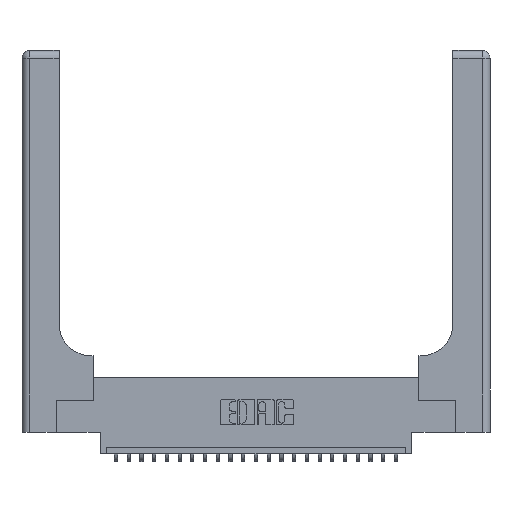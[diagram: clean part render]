
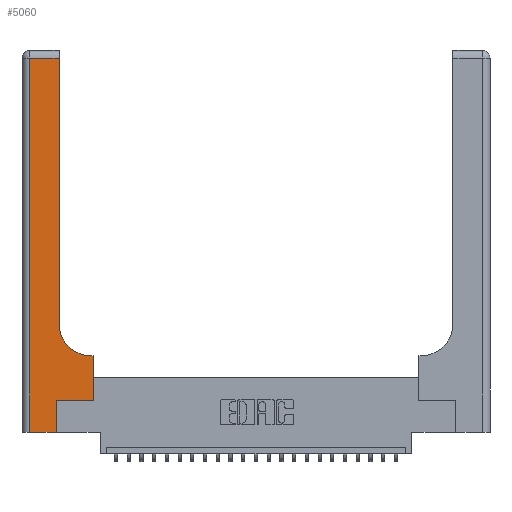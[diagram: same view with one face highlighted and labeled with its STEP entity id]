
A CAD part, top view. The second image highlights one B-rep face of the part: STEP entity #5060.
In plain terms, the highlighted planar face has unit normal (0, 0, 1).
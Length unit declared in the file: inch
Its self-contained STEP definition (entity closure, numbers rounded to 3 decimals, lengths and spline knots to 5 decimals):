
#475 = CARTESIAN_POINT ( 'NONE',  ( 0.269, 0.25, 0.37 ) ) ;
#723 = DIRECTION ( 'NONE',  ( 1., 0., 0. ) ) ;
#1697 = CARTESIAN_POINT ( 'NONE',  ( 0.2915, 3., 0.37 ) ) ;
#2008 = ORIENTED_EDGE ( 'NONE', *, *, #23316, .T. ) ;
#2259 = CARTESIAN_POINT ( 'NONE',  ( 0., 0., 0.37 ) ) ;
#2364 = VERTEX_POINT ( 'NONE', #15380 ) ;
#2484 = EDGE_CURVE ( 'NONE', #16981, #15620, #15268, .T. ) ;
#2587 = VECTOR ( 'NONE', #13204, 39.37008 ) ;
#2593 = LINE ( 'NONE', #14605, #2926 ) ;
#2719 = CARTESIAN_POINT ( 'NONE',  ( 0.06, 3., 0.37 ) ) ;
#2878 = VERTEX_POINT ( 'NONE', #475 ) ;
#2926 = VECTOR ( 'NONE', #5136, 39.37008 ) ;
#3103 = DIRECTION ( 'NONE',  ( -1., 0., 0. ) ) ;
#3133 = DIRECTION ( 'NONE',  ( 0., 0., -1. ) ) ;
#3677 = DIRECTION ( 'NONE',  ( 0., 1., 0. ) ) ;
#3927 = EDGE_CURVE ( 'NONE', #2878, #24777, #5741, .T. ) ;
#4013 = DIRECTION ( 'NONE',  ( -1., 0., 0. ) ) ;
#4089 = VECTOR ( 'NONE', #723, 39.37008 ) ;
#4716 = CARTESIAN_POINT ( 'NONE',  ( 0.06, 2.94, 0.37 ) ) ;
#4819 = AXIS2_PLACEMENT_3D ( 'NONE', #8930, #20790, #3103 ) ;
#5060 = ADVANCED_FACE ( 'NONE', ( #5089 ), #20532, .F. ) ;
#5084 = LINE ( 'NONE', #23223, #7850 ) ;
#5089 = FACE_OUTER_BOUND ( 'NONE', #15781, .T. ) ;
#5136 = DIRECTION ( 'NONE',  ( 0., 1., 0. ) ) ;
#5344 = LINE ( 'NONE', #2259, #4089 ) ;
#5741 = LINE ( 'NONE', #20090, #6657 ) ;
#5994 = VECTOR ( 'NONE', #23192, 39.37008 ) ;
#6182 = EDGE_CURVE ( 'NONE', #15620, #6461, #5344, .T. ) ;
#6461 = VERTEX_POINT ( 'NONE', #20992 ) ;
#6657 = VECTOR ( 'NONE', #23811, 39.37008 ) ;
#6873 = ORIENTED_EDGE ( 'NONE', *, *, #7666, .T. ) ;
#6950 = VERTEX_POINT ( 'NONE', #8498 ) ;
#7040 = CARTESIAN_POINT ( 'NONE',  ( 0.2915, 0.85, 0.37 ) ) ;
#7554 = ORIENTED_EDGE ( 'NONE', *, *, #11364, .T. ) ;
#7666 = EDGE_CURVE ( 'NONE', #19085, #6950, #7728, .T. ) ;
#7728 = LINE ( 'NONE', #1697, #19624 ) ;
#7850 = VECTOR ( 'NONE', #4013, 39.37008 ) ;
#8498 = CARTESIAN_POINT ( 'NONE',  ( 0.2915, 2.94, 0.37 ) ) ;
#8930 = CARTESIAN_POINT ( 'NONE',  ( 0., 3., 0.37 ) ) ;
#9279 = ORIENTED_EDGE ( 'NONE', *, *, #14532, .T. ) ;
#9566 = CARTESIAN_POINT ( 'NONE',  ( 0.269, 0., 0.37 ) ) ;
#10097 = VECTOR ( 'NONE', #18462, 39.37008 ) ;
#11364 = EDGE_CURVE ( 'NONE', #6461, #2878, #21837, .T. ) ;
#11471 = ORIENTED_EDGE ( 'NONE', *, *, #11594, .T. ) ;
#11594 = EDGE_CURVE ( 'NONE', #6950, #16981, #13589, .T. ) ;
#13204 = DIRECTION ( 'NONE',  ( -1., 0., 0. ) ) ;
#13410 = ORIENTED_EDGE ( 'NONE', *, *, #6182, .T. ) ;
#13589 = LINE ( 'NONE', #21007, #2587 ) ;
#14532 = EDGE_CURVE ( 'NONE', #2364, #19539, #5084, .T. ) ;
#14605 = CARTESIAN_POINT ( 'NONE',  ( 0.5585, 0.25, 0.37 ) ) ;
#15268 = LINE ( 'NONE', #2719, #10097 ) ;
#15380 = CARTESIAN_POINT ( 'NONE',  ( 0.5585, 0.6, 0.37 ) ) ;
#15620 = VERTEX_POINT ( 'NONE', #16010 ) ;
#15781 = EDGE_LOOP ( 'NONE', ( #6873, #11471, #17626, #13410, #7554, #18110, #2008, #9279, #23185 ) ) ;
#16010 = CARTESIAN_POINT ( 'NONE',  ( 0.06, 0., 0.37 ) ) ;
#16829 = DIRECTION ( 'NONE',  ( 1., 0., 0. ) ) ;
#16981 = VERTEX_POINT ( 'NONE', #4716 ) ;
#17626 = ORIENTED_EDGE ( 'NONE', *, *, #2484, .T. ) ;
#18110 = ORIENTED_EDGE ( 'NONE', *, *, #3927, .T. ) ;
#18462 = DIRECTION ( 'NONE',  ( 0., -1., 0. ) ) ;
#19085 = VERTEX_POINT ( 'NONE', #7040 ) ;
#19539 = VERTEX_POINT ( 'NONE', #22743 ) ;
#19624 = VECTOR ( 'NONE', #3677, 39.37008 ) ;
#19755 = CARTESIAN_POINT ( 'NONE',  ( 0.5585, 0.25, 0.37 ) ) ;
#20090 = CARTESIAN_POINT ( 'NONE',  ( 0.269, 0.25, 0.37 ) ) ;
#20431 = CIRCLE ( 'NONE', #21790, 0.25 ) ;
#20532 = PLANE ( 'NONE',  #4819 ) ;
#20653 = CARTESIAN_POINT ( 'NONE',  ( 0.5415, 0.85, 0.37 ) ) ;
#20790 = DIRECTION ( 'NONE',  ( 0., 0., -1. ) ) ;
#20992 = CARTESIAN_POINT ( 'NONE',  ( 0.269, 0., 0.37 ) ) ;
#21007 = CARTESIAN_POINT ( 'NONE',  ( 0., 2.94, 0.37 ) ) ;
#21341 = EDGE_CURVE ( 'NONE', #19539, #19085, #20431, .T. ) ;
#21790 = AXIS2_PLACEMENT_3D ( 'NONE', #20653, #3133, #16829 ) ;
#21837 = LINE ( 'NONE', #9566, #5994 ) ;
#22743 = CARTESIAN_POINT ( 'NONE',  ( 0.5415, 0.6, 0.37 ) ) ;
#23185 = ORIENTED_EDGE ( 'NONE', *, *, #21341, .T. ) ;
#23192 = DIRECTION ( 'NONE',  ( 0., 1., 0. ) ) ;
#23223 = CARTESIAN_POINT ( 'NONE',  ( 0.2915, 0.6, 0.37 ) ) ;
#23316 = EDGE_CURVE ( 'NONE', #24777, #2364, #2593, .T. ) ;
#23811 = DIRECTION ( 'NONE',  ( 1., 0., 0. ) ) ;
#24777 = VERTEX_POINT ( 'NONE', #19755 ) ;
